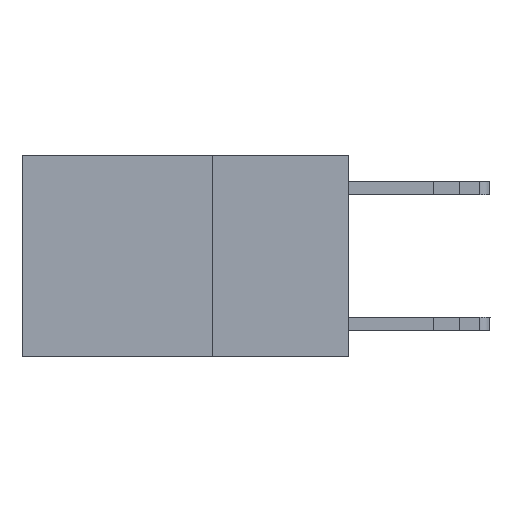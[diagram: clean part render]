
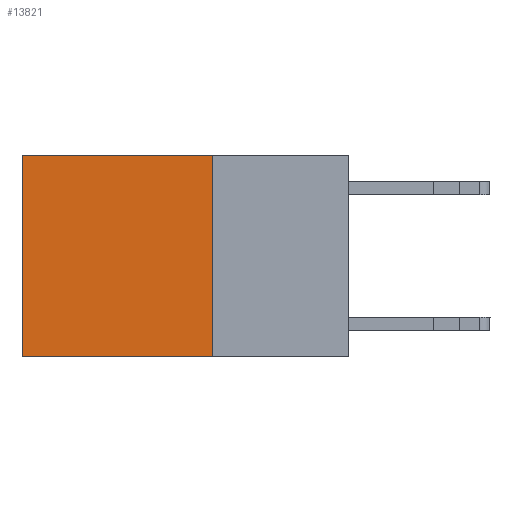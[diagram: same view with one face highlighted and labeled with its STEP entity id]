
A CAD part, left-side view. The second image highlights one B-rep face of the part: STEP entity #13821.
In plain terms, the highlighted planar face has unit normal (-1, 0, 0).
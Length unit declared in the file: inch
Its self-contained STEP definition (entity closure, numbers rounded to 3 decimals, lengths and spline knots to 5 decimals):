
#47 = CARTESIAN_POINT ( 'NONE',  ( 0.2625, 0.6, 0. ) ) ;
#233 = LINE ( 'NONE', #2187, #18907 ) ;
#403 = EDGE_CURVE ( 'NONE', #10246, #4643, #18862, .T. ) ;
#1134 = EDGE_LOOP ( 'NONE', ( #7968, #12672, #18069, #5344 ) ) ;
#1167 = CARTESIAN_POINT ( 'NONE',  ( 0.2625, 0.25, 0. ) ) ;
#1349 = DIRECTION ( 'NONE',  ( 0., 0., -1. ) ) ;
#1410 = CARTESIAN_POINT ( 'NONE',  ( 0.2625, 0.25, -0.37 ) ) ;
#1687 = EDGE_CURVE ( 'NONE', #4643, #11411, #16589, .T. ) ;
#1936 = LINE ( 'NONE', #1410, #4982 ) ;
#2187 = CARTESIAN_POINT ( 'NONE',  ( 0.2625, 0.25, 0. ) ) ;
#4643 = VERTEX_POINT ( 'NONE', #47 ) ;
#4957 = EDGE_CURVE ( 'NONE', #10246, #17369, #233, .T. ) ;
#4982 = VECTOR ( 'NONE', #13310, 39.37008 ) ;
#5344 = ORIENTED_EDGE ( 'NONE', *, *, #403, .T. ) ;
#6011 = FACE_OUTER_BOUND ( 'NONE', #1134, .T. ) ;
#7145 = CARTESIAN_POINT ( 'NONE',  ( 0.2625, 0.6, -0.37 ) ) ;
#7291 = CARTESIAN_POINT ( 'NONE',  ( 0.2625, 0.25, 0. ) ) ;
#7570 = CARTESIAN_POINT ( 'NONE',  ( 0.2625, 0.25, 0. ) ) ;
#7968 = ORIENTED_EDGE ( 'NONE', *, *, #1687, .T. ) ;
#7975 = EDGE_CURVE ( 'NONE', #17369, #11411, #1936, .T. ) ;
#8088 = VECTOR ( 'NONE', #14281, 39.37008 ) ;
#9627 = DIRECTION ( 'NONE',  ( 0., 0., -1. ) ) ;
#9773 = DIRECTION ( 'NONE',  ( 0., 0., -1. ) ) ;
#9799 = CARTESIAN_POINT ( 'NONE',  ( 0.2625, 0.6, 0. ) ) ;
#10246 = VERTEX_POINT ( 'NONE', #7570 ) ;
#10258 = DIRECTION ( 'NONE',  ( 1., 0., 0. ) ) ;
#11411 = VERTEX_POINT ( 'NONE', #7145 ) ;
#12672 = ORIENTED_EDGE ( 'NONE', *, *, #7975, .F. ) ;
#13310 = DIRECTION ( 'NONE',  ( 0., 1., 0. ) ) ;
#13821 = ADVANCED_FACE ( 'NONE', ( #6011 ), #16129, .F. ) ;
#14281 = DIRECTION ( 'NONE',  ( 0., 1., 0. ) ) ;
#16129 = PLANE ( 'NONE',  #18237 ) ;
#16143 = VECTOR ( 'NONE', #9773, 39.37008 ) ;
#16589 = LINE ( 'NONE', #9799, #16143 ) ;
#17369 = VERTEX_POINT ( 'NONE', #17653 ) ;
#17653 = CARTESIAN_POINT ( 'NONE',  ( 0.2625, 0.25, -0.37 ) ) ;
#18069 = ORIENTED_EDGE ( 'NONE', *, *, #4957, .F. ) ;
#18237 = AXIS2_PLACEMENT_3D ( 'NONE', #7291, #10258, #1349 ) ;
#18862 = LINE ( 'NONE', #1167, #8088 ) ;
#18907 = VECTOR ( 'NONE', #9627, 39.37008 ) ;
